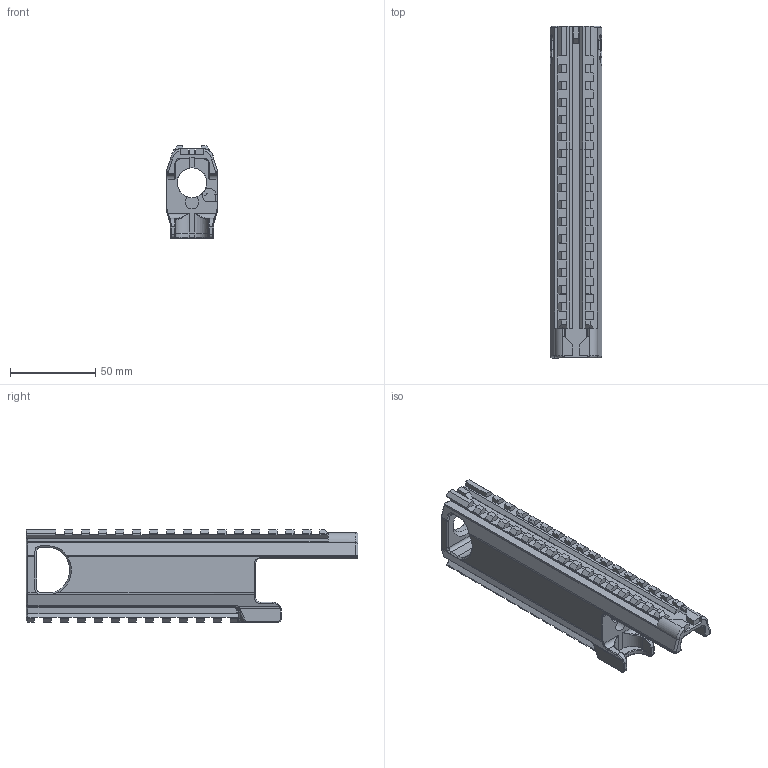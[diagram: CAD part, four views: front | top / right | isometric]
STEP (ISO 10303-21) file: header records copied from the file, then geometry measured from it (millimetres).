
FILE_DESCRIPTION(/* description */ (''),/* implementation_level */ '2;1');
FILE_NAME(/* name */ 'Big Wrangler Railed.step',/* time_stamp */ '2021-09-08T14:22:31-06:00',/* author */ (''),/* organization */ (''),/* preprocessor_version */ 'ST-DEVELOPER v18.1',/* originating_system */ 'Autodesk Translation Framework v10.10.0.1391',/* authorisation */ '');
FILE_SCHEMA (('AUTOMOTIVE_DESIGN { 1 0 10303 214 3 1 1 }'));
Length unit declared in the file: millimetre
Products named in the file (1): Wrangler Mods
Bounding box: 30.48 x 195.2 x 54.29 mm (x, y, z)
Volume: 143297.5 mm3; surface area: 45473.9 mm2
Topology: 1 solids, 1 shells, 734 faces, 1931 edges, 1190 vertices
Faces by surface type: plane 541, cylinder 100, bspline 45, torus 30, cone 16, sphere 2
Full cylindrical faces by diameter (mm): 4 x1, 6.5 x1, 17.5 x2
Entity records: 23324 total; most frequent: CARTESIAN_POINT 5424, ORIENTED_EDGE 3854, DIRECTION 3494, EDGE_CURVE 1927, LINE 1558, VECTOR 1558, VERTEX_POINT 1190, AXIS2_PLACEMENT_3D 968
